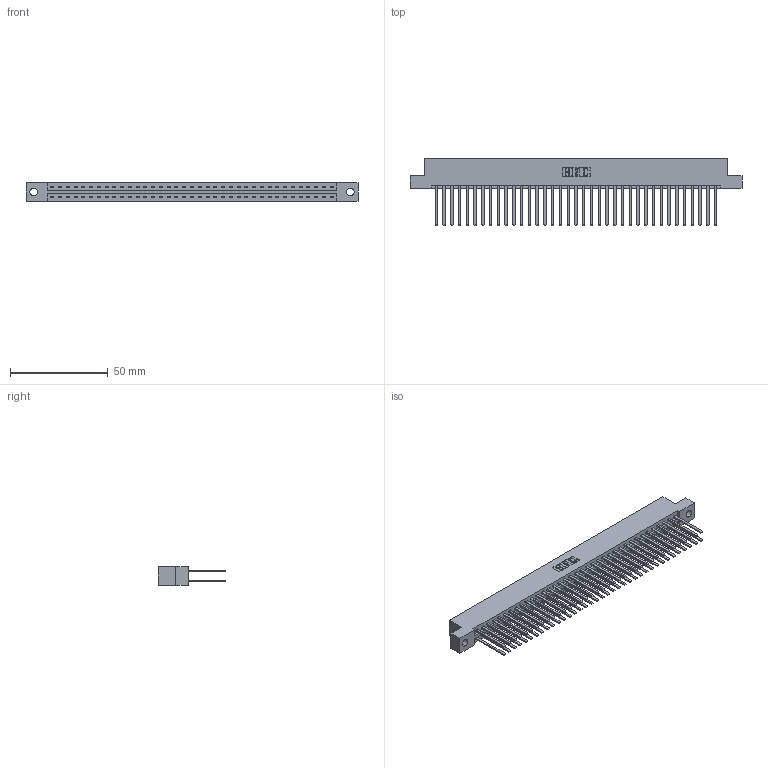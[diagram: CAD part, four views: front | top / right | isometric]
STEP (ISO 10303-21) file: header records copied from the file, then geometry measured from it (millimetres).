
FILE_DESCRIPTION (( 'STEP AP203' ), '1' );
FILE_NAME ('337-074-544-204.STEP', '2018-08-11T17:48:56', ( '' ), ( '' ), 'SwSTEP 2.0', 'SolidWorks 2016', '' );
FILE_SCHEMA (( 'CONFIG_CONTROL_DESIGN' ));
Length unit declared in the file: inch
Products named in the file (3): 337 Part_Flush Mounting Lugs - 0.156 Dia-TH; 345-292-001_345-293-144; 337-074-544-204
Assembly tree (75 placements, depth 2):
  337-074-544-204
    337 Part_Flush Mounting Lugs - 0.156 Dia-TH
    345-292-001_345-293-144  x74
Bounding box: 169.62 x 34.3 x 9.4 mm (x, y, z)
Volume: 18759 mm3; surface area: 24344.6 mm2
Topology: 75 solids, 75 shells, 3666 faces, 10893 edges, 7162 vertices
Faces by surface type: plane 2586, cylinder 1080
Entity records: 29153 total; most frequent: CARTESIAN_POINT 4914, ORIENTED_EDGE 4850, DIRECTION 4185, EDGE_CURVE 2425, VECTOR 2301, LINE 2301, VERTEX_POINT 1614, AXIS2_PLACEMENT_3D 942
